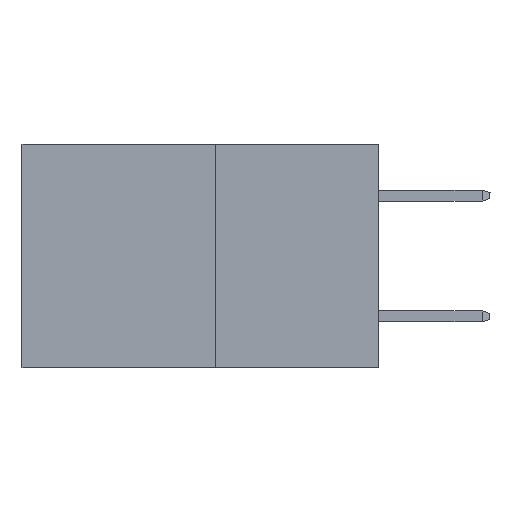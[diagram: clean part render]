
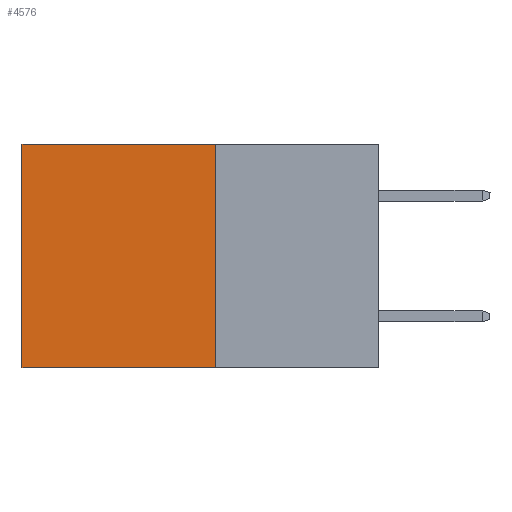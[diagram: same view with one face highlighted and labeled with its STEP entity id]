
A CAD part, left-side view. The second image highlights one B-rep face of the part: STEP entity #4576.
In plain terms, the highlighted planar face has unit normal (-1, 0, 0).
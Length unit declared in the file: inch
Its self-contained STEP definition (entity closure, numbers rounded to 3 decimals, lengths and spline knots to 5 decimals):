
#182 = DIRECTION ( 'NONE',  ( 0., 0., -1. ) ) ;
#352 = DIRECTION ( 'NONE',  ( 0., 0., -1. ) ) ;
#613 = EDGE_LOOP ( 'NONE', ( #8588, #1182, #5935, #1155 ) ) ;
#894 = VERTEX_POINT ( 'NONE', #3366 ) ;
#1155 = ORIENTED_EDGE ( 'NONE', *, *, #3332, .T. ) ;
#1182 = ORIENTED_EDGE ( 'NONE', *, *, #10298, .F. ) ;
#2200 = VERTEX_POINT ( 'NONE', #4367 ) ;
#2791 = AXIS2_PLACEMENT_3D ( 'NONE', #3992, #5777, #352 ) ;
#2837 = CARTESIAN_POINT ( 'NONE',  ( 0.277, 0.59, -0.37 ) ) ;
#2900 = CARTESIAN_POINT ( 'NONE',  ( 0.277, 0.27, 0. ) ) ;
#2913 = DIRECTION ( 'NONE',  ( 0., 1., 0. ) ) ;
#3117 = VECTOR ( 'NONE', #182, 39.37008 ) ;
#3332 = EDGE_CURVE ( 'NONE', #894, #2200, #8189, .T. ) ;
#3366 = CARTESIAN_POINT ( 'NONE',  ( 0.277, 0.27, 0. ) ) ;
#3662 = DIRECTION ( 'NONE',  ( 0., 1., 0. ) ) ;
#3992 = CARTESIAN_POINT ( 'NONE',  ( 0.277, 0.27, -0.37 ) ) ;
#4314 = CARTESIAN_POINT ( 'NONE',  ( 0.277, 0.27, -0.37 ) ) ;
#4367 = CARTESIAN_POINT ( 'NONE',  ( 0.277, 0.59, 0. ) ) ;
#4576 = ADVANCED_FACE ( 'NONE', ( #5919 ), #11158, .F. ) ;
#4626 = VECTOR ( 'NONE', #6546, 39.37008 ) ;
#4672 = VECTOR ( 'NONE', #2913, 39.37008 ) ;
#4904 = VECTOR ( 'NONE', #3662, 39.37008 ) ;
#4907 = LINE ( 'NONE', #8373, #4626 ) ;
#5766 = EDGE_CURVE ( 'NONE', #2200, #9127, #8414, .T. ) ;
#5777 = DIRECTION ( 'NONE',  ( 1., 0., 0. ) ) ;
#5817 = EDGE_CURVE ( 'NONE', #894, #10841, #4907, .T. ) ;
#5919 = FACE_OUTER_BOUND ( 'NONE', #613, .T. ) ;
#5935 = ORIENTED_EDGE ( 'NONE', *, *, #5817, .F. ) ;
#6546 = DIRECTION ( 'NONE',  ( 0., 0., -1. ) ) ;
#7012 = LINE ( 'NONE', #9000, #4904 ) ;
#8189 = LINE ( 'NONE', #2900, #4672 ) ;
#8373 = CARTESIAN_POINT ( 'NONE',  ( 0.277, 0.27, -0.37 ) ) ;
#8414 = LINE ( 'NONE', #11025, #3117 ) ;
#8588 = ORIENTED_EDGE ( 'NONE', *, *, #5766, .T. ) ;
#9000 = CARTESIAN_POINT ( 'NONE',  ( 0.277, 0.27, -0.37 ) ) ;
#9127 = VERTEX_POINT ( 'NONE', #2837 ) ;
#10298 = EDGE_CURVE ( 'NONE', #10841, #9127, #7012, .T. ) ;
#10841 = VERTEX_POINT ( 'NONE', #4314 ) ;
#11025 = CARTESIAN_POINT ( 'NONE',  ( 0.277, 0.59, -0.37 ) ) ;
#11158 = PLANE ( 'NONE',  #2791 ) ;
